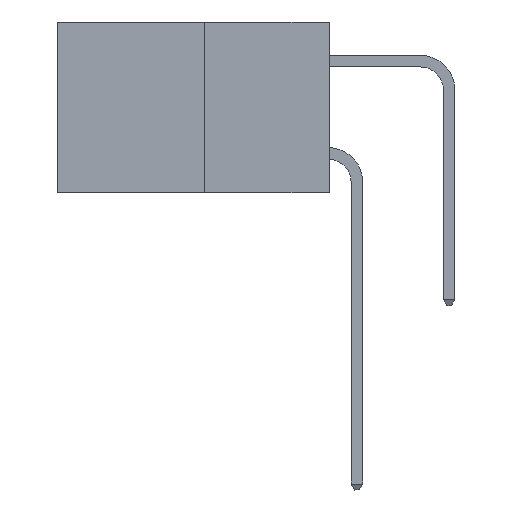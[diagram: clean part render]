
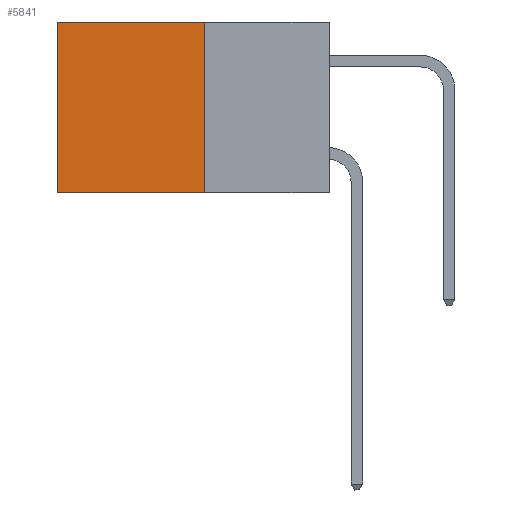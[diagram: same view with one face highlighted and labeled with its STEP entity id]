
A CAD part, left-side view. The second image highlights one B-rep face of the part: STEP entity #5841.
In plain terms, the highlighted planar face has unit normal (-1, 0, 0).
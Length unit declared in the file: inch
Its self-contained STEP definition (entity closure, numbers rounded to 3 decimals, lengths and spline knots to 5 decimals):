
#2 = DIRECTION ( 'NONE',  ( 0., 1., 0. ) ) ;
#46 = CARTESIAN_POINT ( 'NONE',  ( 0.277, 0.27, 0. ) ) ;
#62 = VERTEX_POINT ( 'NONE', #6586 ) ;
#197 = CARTESIAN_POINT ( 'NONE',  ( 0.277, 0.27, -0.37 ) ) ;
#343 = DIRECTION ( 'NONE',  ( 0., 1., 0. ) ) ;
#1788 = EDGE_CURVE ( 'NONE', #12108, #62, #4040, .T. ) ;
#1844 = PLANE ( 'NONE',  #12088 ) ;
#1972 = CARTESIAN_POINT ( 'NONE',  ( 0.277, 0.59, 0. ) ) ;
#2075 = VECTOR ( 'NONE', #343, 39.37008 ) ;
#2897 = ORIENTED_EDGE ( 'NONE', *, *, #5124, .T. ) ;
#2909 = ORIENTED_EDGE ( 'NONE', *, *, #4859, .F. ) ;
#2924 = ORIENTED_EDGE ( 'NONE', *, *, #1788, .F. ) ;
#2935 = ORIENTED_EDGE ( 'NONE', *, *, #4862, .T. ) ;
#3335 = CARTESIAN_POINT ( 'NONE',  ( 0.277, 0.27, 0. ) ) ;
#3631 = CARTESIAN_POINT ( 'NONE',  ( 0.277, 0.59, -0.37 ) ) ;
#4040 = LINE ( 'NONE', #8990, #8891 ) ;
#4802 = VERTEX_POINT ( 'NONE', #1972 ) ;
#4859 = EDGE_CURVE ( 'NONE', #62, #6607, #12124, .T. ) ;
#4862 = EDGE_CURVE ( 'NONE', #12108, #4802, #9822, .T. ) ;
#4966 = CARTESIAN_POINT ( 'NONE',  ( 0.277, 0.27, -0.37 ) ) ;
#5124 = EDGE_CURVE ( 'NONE', #4802, #6607, #8066, .T. ) ;
#5125 = VECTOR ( 'NONE', #11236, 39.37008 ) ;
#5841 = ADVANCED_FACE ( 'NONE', ( #8735 ), #1844, .F. ) ;
#6007 = DIRECTION ( 'NONE',  ( 0., 0., -1. ) ) ;
#6586 = CARTESIAN_POINT ( 'NONE',  ( 0.277, 0.27, -0.37 ) ) ;
#6607 = VERTEX_POINT ( 'NONE', #3631 ) ;
#8066 = LINE ( 'NONE', #9605, #5125 ) ;
#8735 = FACE_OUTER_BOUND ( 'NONE', #10939, .T. ) ;
#8891 = VECTOR ( 'NONE', #8957, 39.37008 ) ;
#8957 = DIRECTION ( 'NONE',  ( 0., 0., -1. ) ) ;
#8990 = CARTESIAN_POINT ( 'NONE',  ( 0.277, 0.27, -0.37 ) ) ;
#9599 = VECTOR ( 'NONE', #2, 39.37008 ) ;
#9605 = CARTESIAN_POINT ( 'NONE',  ( 0.277, 0.59, -0.37 ) ) ;
#9822 = LINE ( 'NONE', #46, #9599 ) ;
#10939 = EDGE_LOOP ( 'NONE', ( #2897, #2909, #2924, #2935 ) ) ;
#11236 = DIRECTION ( 'NONE',  ( 0., 0., -1. ) ) ;
#11399 = DIRECTION ( 'NONE',  ( 1., 0., 0. ) ) ;
#12088 = AXIS2_PLACEMENT_3D ( 'NONE', #4966, #11399, #6007 ) ;
#12108 = VERTEX_POINT ( 'NONE', #3335 ) ;
#12124 = LINE ( 'NONE', #197, #2075 ) ;
